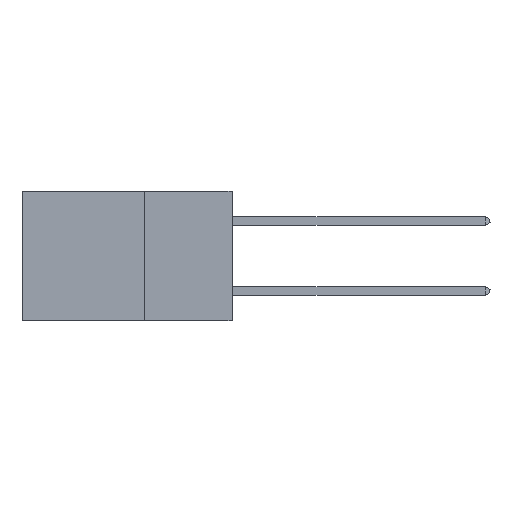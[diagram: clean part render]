
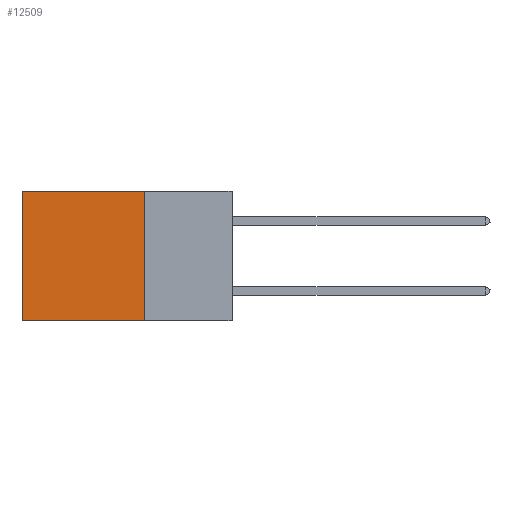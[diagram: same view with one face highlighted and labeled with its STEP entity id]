
A CAD part, left-side view. The second image highlights one B-rep face of the part: STEP entity #12509.
In plain terms, the highlighted planar face has unit normal (-1, 0, 0).
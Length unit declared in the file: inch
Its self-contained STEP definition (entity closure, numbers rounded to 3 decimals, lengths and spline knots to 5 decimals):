
#829 = EDGE_CURVE ( 'NONE', #11204, #10871, #3953, .T. ) ;
#2515 = LINE ( 'NONE', #2637, #18754 ) ;
#2636 = CARTESIAN_POINT ( 'NONE',  ( 0.2875, 0.25, 0. ) ) ;
#2637 = CARTESIAN_POINT ( 'NONE',  ( 0.2875, 0.25, 0. ) ) ;
#3145 = EDGE_CURVE ( 'NONE', #14635, #10762, #4367, .T. ) ;
#3905 = VECTOR ( 'NONE', #7283, 39.37008 ) ;
#3953 = LINE ( 'NONE', #12545, #18955 ) ;
#4309 = ORIENTED_EDGE ( 'NONE', *, *, #10907, .F. ) ;
#4367 = LINE ( 'NONE', #7035, #3905 ) ;
#4556 = CARTESIAN_POINT ( 'NONE',  ( 0.2875, 0.6, -0.37 ) ) ;
#5384 = ORIENTED_EDGE ( 'NONE', *, *, #829, .F. ) ;
#5818 = FACE_OUTER_BOUND ( 'NONE', #8621, .T. ) ;
#6734 = ORIENTED_EDGE ( 'NONE', *, *, #3145, .T. ) ;
#7035 = CARTESIAN_POINT ( 'NONE',  ( 0.2875, 0.6, 0. ) ) ;
#7283 = DIRECTION ( 'NONE',  ( 0., 0., -1. ) ) ;
#7303 = EDGE_CURVE ( 'NONE', #11204, #14635, #2515, .T. ) ;
#7610 = CARTESIAN_POINT ( 'NONE',  ( 0.2875, 0.25, 0. ) ) ;
#8621 = EDGE_LOOP ( 'NONE', ( #6734, #4309, #5384, #14525 ) ) ;
#8842 = CARTESIAN_POINT ( 'NONE',  ( 0.2875, 0.6, 0. ) ) ;
#9487 = CARTESIAN_POINT ( 'NONE',  ( 0.2875, 0.25, -0.37 ) ) ;
#10419 = AXIS2_PLACEMENT_3D ( 'NONE', #7610, #19211, #10663 ) ;
#10663 = DIRECTION ( 'NONE',  ( 0., 0., -1. ) ) ;
#10762 = VERTEX_POINT ( 'NONE', #4556 ) ;
#10871 = VERTEX_POINT ( 'NONE', #9487 ) ;
#10907 = EDGE_CURVE ( 'NONE', #10871, #10762, #19161, .T. ) ;
#11204 = VERTEX_POINT ( 'NONE', #2636 ) ;
#12509 = ADVANCED_FACE ( 'NONE', ( #5818 ), #17780, .F. ) ;
#12545 = CARTESIAN_POINT ( 'NONE',  ( 0.2875, 0.25, 0. ) ) ;
#12660 = DIRECTION ( 'NONE',  ( 0., 0., -1. ) ) ;
#13233 = DIRECTION ( 'NONE',  ( 0., 1., 0. ) ) ;
#14525 = ORIENTED_EDGE ( 'NONE', *, *, #7303, .T. ) ;
#14635 = VERTEX_POINT ( 'NONE', #8842 ) ;
#15388 = VECTOR ( 'NONE', #16773, 39.37008 ) ;
#16773 = DIRECTION ( 'NONE',  ( 0., 1., 0. ) ) ;
#17780 = PLANE ( 'NONE',  #10419 ) ;
#18088 = CARTESIAN_POINT ( 'NONE',  ( 0.2875, 0.25, -0.37 ) ) ;
#18754 = VECTOR ( 'NONE', #13233, 39.37008 ) ;
#18955 = VECTOR ( 'NONE', #12660, 39.37008 ) ;
#19161 = LINE ( 'NONE', #18088, #15388 ) ;
#19211 = DIRECTION ( 'NONE',  ( 1., 0., 0. ) ) ;
